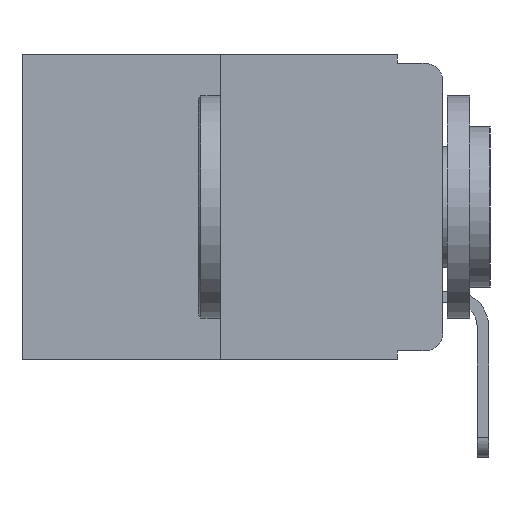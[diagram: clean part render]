
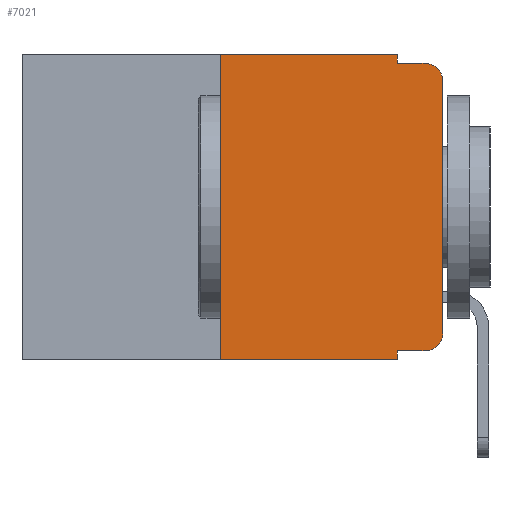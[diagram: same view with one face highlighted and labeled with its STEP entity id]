
A CAD part, left-side view. The second image highlights one B-rep face of the part: STEP entity #7021.
In plain terms, the highlighted planar face has unit normal (-1, 0, 0).
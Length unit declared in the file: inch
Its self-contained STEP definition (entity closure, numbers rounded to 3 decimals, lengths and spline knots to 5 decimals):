
#167 = CARTESIAN_POINT ( 'NONE',  ( 0., 0.02, -0.01 ) ) ;
#534 = PLANE ( 'NONE',  #9916 ) ;
#698 = DIRECTION ( 'NONE',  ( 0., -1., 0. ) ) ;
#748 = VECTOR ( 'NONE', #11273, 39.37008 ) ;
#861 = DIRECTION ( 'NONE',  ( 0., -1., 0. ) ) ;
#1064 = VERTEX_POINT ( 'NONE', #2442 ) ;
#1119 = VERTEX_POINT ( 'NONE', #3418 ) ;
#1237 = VECTOR ( 'NONE', #861, 39.37008 ) ;
#1361 = ORIENTED_EDGE ( 'NONE', *, *, #3174, .F. ) ;
#1393 = LINE ( 'NONE', #10294, #748 ) ;
#2442 = CARTESIAN_POINT ( 'NONE',  ( 0., 0.051, -0.333 ) ) ;
#2494 = DIRECTION ( 'NONE',  ( 0., 0., -1. ) ) ;
#2503 = EDGE_CURVE ( 'NONE', #12181, #12278, #12538, .T. ) ;
#2567 = DIRECTION ( 'NONE',  ( 0., 0., -1. ) ) ;
#2660 = DIRECTION ( 'NONE',  ( 0., 0., 1. ) ) ;
#2830 = CARTESIAN_POINT ( 'NONE',  ( 0., 0.473, 0. ) ) ;
#2944 = CARTESIAN_POINT ( 'NONE',  ( 0., 0.02, -0.03 ) ) ;
#2983 = EDGE_CURVE ( 'NONE', #7299, #12175, #6538, .T. ) ;
#3170 = EDGE_LOOP ( 'NONE', ( #11656, #5457, #12058, #1361, #3819, #6352, #10543, #3586, #12664, #11958 ) ) ;
#3174 = EDGE_CURVE ( 'NONE', #6424, #7299, #5552, .T. ) ;
#3418 = CARTESIAN_POINT ( 'NONE',  ( 0., 0.25, -0.343 ) ) ;
#3443 = LINE ( 'NONE', #6551, #9406 ) ;
#3541 = EDGE_CURVE ( 'NONE', #1064, #12181, #12509, .T. ) ;
#3586 = ORIENTED_EDGE ( 'NONE', *, *, #7507, .F. ) ;
#3664 = DIRECTION ( 'NONE',  ( 0., 0., -1. ) ) ;
#3705 = VECTOR ( 'NONE', #6351, 39.37008 ) ;
#3716 = CARTESIAN_POINT ( 'NONE',  ( 0., 0.25, 0. ) ) ;
#3819 = ORIENTED_EDGE ( 'NONE', *, *, #6891, .F. ) ;
#3885 = VECTOR ( 'NONE', #2567, 39.37008 ) ;
#4036 = CARTESIAN_POINT ( 'NONE',  ( 0., 0.051, -0.01 ) ) ;
#4504 = CARTESIAN_POINT ( 'NONE',  ( 0., 0.051, 0. ) ) ;
#5057 = VERTEX_POINT ( 'NONE', #11127 ) ;
#5189 = VECTOR ( 'NONE', #2494, 39.37008 ) ;
#5215 = CARTESIAN_POINT ( 'NONE',  ( 0., 0.051, -0.01 ) ) ;
#5382 = VERTEX_POINT ( 'NONE', #13291 ) ;
#5457 = ORIENTED_EDGE ( 'NONE', *, *, #7257, .T. ) ;
#5552 = LINE ( 'NONE', #4504, #3885 ) ;
#5868 = LINE ( 'NONE', #2830, #12514 ) ;
#6351 = DIRECTION ( 'NONE',  ( 0., -1., 0. ) ) ;
#6352 = ORIENTED_EDGE ( 'NONE', *, *, #12692, .F. ) ;
#6424 = VERTEX_POINT ( 'NONE', #13543 ) ;
#6478 = LINE ( 'NONE', #12283, #9301 ) ;
#6538 = LINE ( 'NONE', #5215, #1237 ) ;
#6551 = CARTESIAN_POINT ( 'NONE',  ( 0., 0., 0. ) ) ;
#6891 = EDGE_CURVE ( 'NONE', #6952, #6424, #5868, .T. ) ;
#6952 = VERTEX_POINT ( 'NONE', #3716 ) ;
#7021 = ADVANCED_FACE ( 'NONE', ( #11497 ), #534, .F. ) ;
#7074 = EDGE_CURVE ( 'NONE', #1119, #5382, #1393, .T. ) ;
#7257 = EDGE_CURVE ( 'NONE', #5057, #12175, #11000, .T. ) ;
#7291 = AXIS2_PLACEMENT_3D ( 'NONE', #2944, #12530, #10338 ) ;
#7299 = VERTEX_POINT ( 'NONE', #4036 ) ;
#7339 = CARTESIAN_POINT ( 'NONE',  ( 0., 0.051, -0.333 ) ) ;
#7401 = AXIS2_PLACEMENT_3D ( 'NONE', #8176, #8255, #10780 ) ;
#7507 = EDGE_CURVE ( 'NONE', #1064, #5382, #8517, .T. ) ;
#8176 = CARTESIAN_POINT ( 'NONE',  ( 0., 0.02, -0.313 ) ) ;
#8255 = DIRECTION ( 'NONE',  ( -1., 0., 0. ) ) ;
#8261 = DIRECTION ( 'NONE',  ( 0., 0., 1. ) ) ;
#8517 = LINE ( 'NONE', #8756, #5189 ) ;
#8756 = CARTESIAN_POINT ( 'NONE',  ( 0., 0.051, 0. ) ) ;
#9301 = VECTOR ( 'NONE', #8261, 39.37008 ) ;
#9325 = EDGE_CURVE ( 'NONE', #12278, #5057, #3443, .T. ) ;
#9406 = VECTOR ( 'NONE', #2660, 39.37008 ) ;
#9916 = AXIS2_PLACEMENT_3D ( 'NONE', #9919, #12210, #3664 ) ;
#9919 = CARTESIAN_POINT ( 'NONE',  ( 0., 0.473, 0. ) ) ;
#10294 = CARTESIAN_POINT ( 'NONE',  ( 0., 0.473, -0.343 ) ) ;
#10338 = DIRECTION ( 'NONE',  ( 0., 0., -1. ) ) ;
#10543 = ORIENTED_EDGE ( 'NONE', *, *, #7074, .T. ) ;
#10780 = DIRECTION ( 'NONE',  ( 0., 0., -1. ) ) ;
#10789 = CARTESIAN_POINT ( 'NONE',  ( 0., 0.02, -0.333 ) ) ;
#11000 = CIRCLE ( 'NONE', #7291, 0.02 ) ;
#11074 = CARTESIAN_POINT ( 'NONE',  ( 0., 0., -0.313 ) ) ;
#11127 = CARTESIAN_POINT ( 'NONE',  ( 0., 0., -0.03 ) ) ;
#11273 = DIRECTION ( 'NONE',  ( 0., -1., 0. ) ) ;
#11497 = FACE_OUTER_BOUND ( 'NONE', #3170, .T. ) ;
#11656 = ORIENTED_EDGE ( 'NONE', *, *, #9325, .T. ) ;
#11958 = ORIENTED_EDGE ( 'NONE', *, *, #2503, .T. ) ;
#12058 = ORIENTED_EDGE ( 'NONE', *, *, #2983, .F. ) ;
#12175 = VERTEX_POINT ( 'NONE', #167 ) ;
#12181 = VERTEX_POINT ( 'NONE', #10789 ) ;
#12210 = DIRECTION ( 'NONE',  ( 1., 0., 0. ) ) ;
#12278 = VERTEX_POINT ( 'NONE', #11074 ) ;
#12283 = CARTESIAN_POINT ( 'NONE',  ( 0., 0.25, 0. ) ) ;
#12509 = LINE ( 'NONE', #7339, #3705 ) ;
#12514 = VECTOR ( 'NONE', #698, 39.37008 ) ;
#12530 = DIRECTION ( 'NONE',  ( -1., 0., 0. ) ) ;
#12538 = CIRCLE ( 'NONE', #7401, 0.02 ) ;
#12664 = ORIENTED_EDGE ( 'NONE', *, *, #3541, .T. ) ;
#12692 = EDGE_CURVE ( 'NONE', #1119, #6952, #6478, .T. ) ;
#13291 = CARTESIAN_POINT ( 'NONE',  ( 0., 0.051, -0.343 ) ) ;
#13543 = CARTESIAN_POINT ( 'NONE',  ( 0., 0.051, 0. ) ) ;
